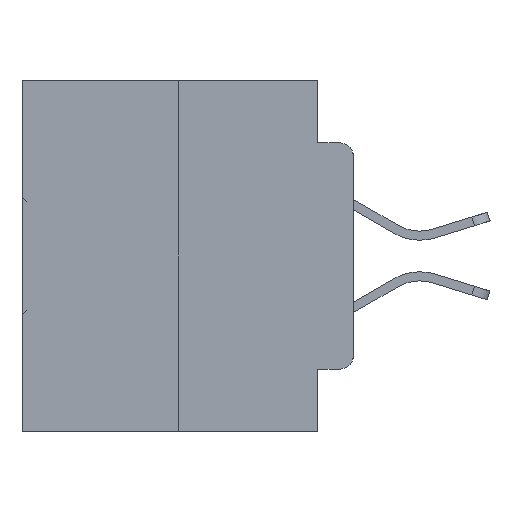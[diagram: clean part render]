
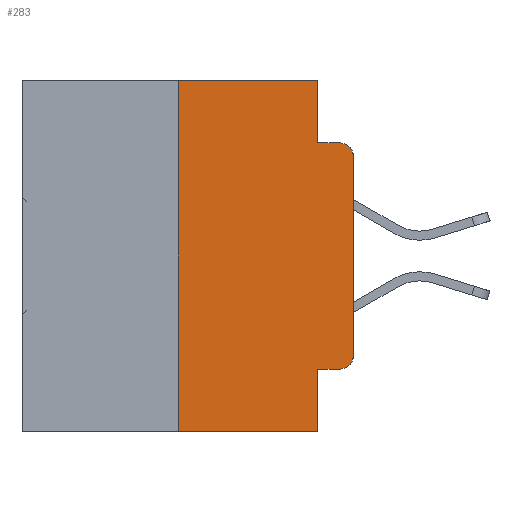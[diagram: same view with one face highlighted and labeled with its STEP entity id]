
A CAD part, left-side view. The second image highlights one B-rep face of the part: STEP entity #283.
In plain terms, the highlighted planar face has unit normal (-1, 0, 0).
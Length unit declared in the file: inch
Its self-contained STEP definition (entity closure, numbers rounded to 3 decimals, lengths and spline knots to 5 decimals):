
#283 = ADVANCED_FACE ( 'NONE', ( #936 ), #9209, .F. ) ;
#379 = CIRCLE ( 'NONE', #20780, 0.02 ) ;
#721 = DIRECTION ( 'NONE',  ( -1., 0., 0. ) ) ;
#795 = CARTESIAN_POINT ( 'NONE',  ( 0., 0., -0.1085 ) ) ;
#884 = DIRECTION ( 'NONE',  ( 0., 0., -1. ) ) ;
#936 = FACE_OUTER_BOUND ( 'NONE', #12232, .T. ) ;
#1084 = VERTEX_POINT ( 'NONE', #8453 ) ;
#2455 = VERTEX_POINT ( 'NONE', #23299 ) ;
#2874 = CARTESIAN_POINT ( 'NONE',  ( 0., 0.473, 0. ) ) ;
#3401 = CARTESIAN_POINT ( 'NONE',  ( 0., 0.25, 0. ) ) ;
#3741 = EDGE_CURVE ( 'NONE', #19938, #26092, #23588, .T. ) ;
#3850 = ORIENTED_EDGE ( 'NONE', *, *, #30058, .F. ) ;
#4195 = VERTEX_POINT ( 'NONE', #8176 ) ;
#4319 = ORIENTED_EDGE ( 'NONE', *, *, #4750, .T. ) ;
#4431 = CARTESIAN_POINT ( 'NONE',  ( 0., 0.051, 0. ) ) ;
#4750 = EDGE_CURVE ( 'NONE', #9382, #9158, #19362, .T. ) ;
#4783 = CARTESIAN_POINT ( 'NONE',  ( 0., 0., -0.3915 ) ) ;
#5505 = ORIENTED_EDGE ( 'NONE', *, *, #3741, .T. ) ;
#6081 = CARTESIAN_POINT ( 'NONE',  ( 0., 0.02, -0.3915 ) ) ;
#6720 = VECTOR ( 'NONE', #14645, 39.37008 ) ;
#7825 = VECTOR ( 'NONE', #33177, 39.37008 ) ;
#8107 = CARTESIAN_POINT ( 'NONE',  ( 0., 0.051, -0.5 ) ) ;
#8176 = CARTESIAN_POINT ( 'NONE',  ( 0., 0.25, 0. ) ) ;
#8453 = CARTESIAN_POINT ( 'NONE',  ( 0., 0.051, -0.0885 ) ) ;
#8735 = DIRECTION ( 'NONE',  ( 0., 0., 1. ) ) ;
#8753 = VERTEX_POINT ( 'NONE', #8107 ) ;
#8771 = EDGE_CURVE ( 'NONE', #15276, #9382, #10706, .T. ) ;
#9158 = VERTEX_POINT ( 'NONE', #10836 ) ;
#9209 = PLANE ( 'NONE',  #10040 ) ;
#9382 = VERTEX_POINT ( 'NONE', #795 ) ;
#9591 = ORIENTED_EDGE ( 'NONE', *, *, #18132, .F. ) ;
#10040 = AXIS2_PLACEMENT_3D ( 'NONE', #27509, #30069, #19752 ) ;
#10706 = LINE ( 'NONE', #16238, #15250 ) ;
#10836 = CARTESIAN_POINT ( 'NONE',  ( 0., 0.02, -0.0885 ) ) ;
#11033 = DIRECTION ( 'NONE',  ( -1., 0., 0. ) ) ;
#11196 = DIRECTION ( 'NONE',  ( 0., 0., -1. ) ) ;
#11705 = LINE ( 'NONE', #27583, #6720 ) ;
#11940 = VECTOR ( 'NONE', #884, 39.37008 ) ;
#12232 = EDGE_LOOP ( 'NONE', ( #14103, #4319, #3850, #26652, #30587, #9591, #29456, #15821, #5505, #17358 ) ) ;
#13827 = VECTOR ( 'NONE', #26167, 39.37008 ) ;
#13846 = EDGE_CURVE ( 'NONE', #2455, #8753, #28721, .T. ) ;
#14103 = ORIENTED_EDGE ( 'NONE', *, *, #8771, .T. ) ;
#14122 = LINE ( 'NONE', #19134, #15883 ) ;
#14293 = DIRECTION ( 'NONE',  ( 0., 0., -1. ) ) ;
#14645 = DIRECTION ( 'NONE',  ( 0., -1., 0. ) ) ;
#15250 = VECTOR ( 'NONE', #21229, 39.37008 ) ;
#15276 = VERTEX_POINT ( 'NONE', #4783 ) ;
#15481 = DIRECTION ( 'NONE',  ( 0., -1., 0. ) ) ;
#15483 = CARTESIAN_POINT ( 'NONE',  ( 0., 0.051, -0.4115 ) ) ;
#15564 = CARTESIAN_POINT ( 'NONE',  ( 0., 0.051, -0.4115 ) ) ;
#15821 = ORIENTED_EDGE ( 'NONE', *, *, #22981, .F. ) ;
#15883 = VECTOR ( 'NONE', #14293, 39.37008 ) ;
#16012 = LINE ( 'NONE', #2874, #33914 ) ;
#16238 = CARTESIAN_POINT ( 'NONE',  ( 0., 0., 0. ) ) ;
#16531 = LINE ( 'NONE', #3401, #27787 ) ;
#17121 = LINE ( 'NONE', #19703, #11940 ) ;
#17358 = ORIENTED_EDGE ( 'NONE', *, *, #22945, .T. ) ;
#18132 = EDGE_CURVE ( 'NONE', #2455, #4195, #16531, .T. ) ;
#18293 = CARTESIAN_POINT ( 'NONE',  ( 0., 0.02, -0.1085 ) ) ;
#19134 = CARTESIAN_POINT ( 'NONE',  ( 0., 0.051, 0. ) ) ;
#19362 = CIRCLE ( 'NONE', #20440, 0.02 ) ;
#19703 = CARTESIAN_POINT ( 'NONE',  ( 0., 0.051, 0. ) ) ;
#19752 = DIRECTION ( 'NONE',  ( 0., 0., -1. ) ) ;
#19938 = VERTEX_POINT ( 'NONE', #15564 ) ;
#20440 = AXIS2_PLACEMENT_3D ( 'NONE', #18293, #11033, #11196 ) ;
#20780 = AXIS2_PLACEMENT_3D ( 'NONE', #6081, #721, #27136 ) ;
#21108 = EDGE_CURVE ( 'NONE', #4195, #25312, #16012, .T. ) ;
#21229 = DIRECTION ( 'NONE',  ( 0., 0., 1. ) ) ;
#22101 = EDGE_CURVE ( 'NONE', #25312, #1084, #14122, .T. ) ;
#22695 = CARTESIAN_POINT ( 'NONE',  ( 0., 0.473, -0.5 ) ) ;
#22945 = EDGE_CURVE ( 'NONE', #26092, #15276, #379, .T. ) ;
#22981 = EDGE_CURVE ( 'NONE', #19938, #8753, #17121, .T. ) ;
#23299 = CARTESIAN_POINT ( 'NONE',  ( 0., 0.25, -0.5 ) ) ;
#23588 = LINE ( 'NONE', #15483, #13827 ) ;
#25178 = CARTESIAN_POINT ( 'NONE',  ( 0., 0.02, -0.4115 ) ) ;
#25312 = VERTEX_POINT ( 'NONE', #4431 ) ;
#26092 = VERTEX_POINT ( 'NONE', #25178 ) ;
#26167 = DIRECTION ( 'NONE',  ( 0., -1., 0. ) ) ;
#26652 = ORIENTED_EDGE ( 'NONE', *, *, #22101, .F. ) ;
#27136 = DIRECTION ( 'NONE',  ( 0., 0., -1. ) ) ;
#27509 = CARTESIAN_POINT ( 'NONE',  ( 0., 0.473, 0. ) ) ;
#27583 = CARTESIAN_POINT ( 'NONE',  ( 0., 0.051, -0.0885 ) ) ;
#27787 = VECTOR ( 'NONE', #8735, 39.37008 ) ;
#28721 = LINE ( 'NONE', #22695, #7825 ) ;
#29456 = ORIENTED_EDGE ( 'NONE', *, *, #13846, .T. ) ;
#30058 = EDGE_CURVE ( 'NONE', #1084, #9158, #11705, .T. ) ;
#30069 = DIRECTION ( 'NONE',  ( 1., 0., 0. ) ) ;
#30587 = ORIENTED_EDGE ( 'NONE', *, *, #21108, .F. ) ;
#33177 = DIRECTION ( 'NONE',  ( 0., -1., 0. ) ) ;
#33914 = VECTOR ( 'NONE', #15481, 39.37008 ) ;
